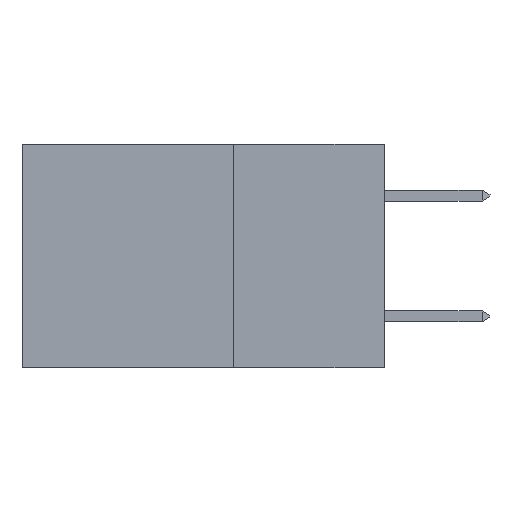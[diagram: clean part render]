
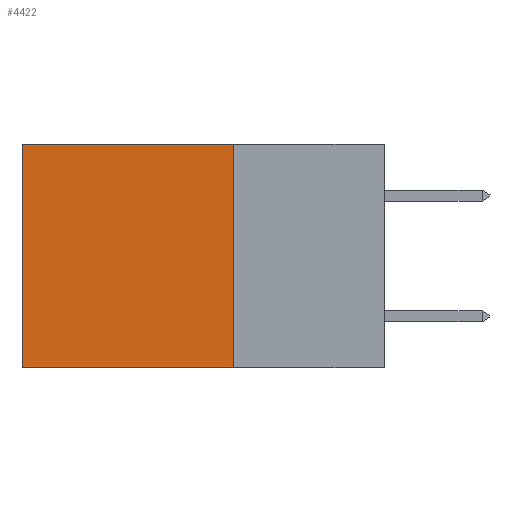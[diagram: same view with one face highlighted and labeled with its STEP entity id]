
A CAD part, left-side view. The second image highlights one B-rep face of the part: STEP entity #4422.
In plain terms, the highlighted planar face has unit normal (-1, 0, 0).
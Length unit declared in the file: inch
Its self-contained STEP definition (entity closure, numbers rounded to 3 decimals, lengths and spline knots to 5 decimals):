
#232 = CARTESIAN_POINT ( 'NONE',  ( 0.2875, 0.25, -0.37 ) ) ;
#830 = CARTESIAN_POINT ( 'NONE',  ( 0.2875, 0.6, 0. ) ) ;
#1557 = LINE ( 'NONE', #14088, #9302 ) ;
#1835 = EDGE_CURVE ( 'NONE', #6135, #8410, #2078, .T. ) ;
#2078 = LINE ( 'NONE', #830, #11527 ) ;
#2556 = ORIENTED_EDGE ( 'NONE', *, *, #1835, .T. ) ;
#2868 = DIRECTION ( 'NONE',  ( 0., 0., -1. ) ) ;
#3298 = ORIENTED_EDGE ( 'NONE', *, *, #4329, .F. ) ;
#4329 = EDGE_CURVE ( 'NONE', #14546, #8410, #8796, .T. ) ;
#4339 = CARTESIAN_POINT ( 'NONE',  ( 0.2875, 0.6, 0. ) ) ;
#4422 = ADVANCED_FACE ( 'NONE', ( #13824 ), #9104, .F. ) ;
#5185 = EDGE_CURVE ( 'NONE', #7229, #6135, #10296, .T. ) ;
#5516 = VECTOR ( 'NONE', #15006, 39.37008 ) ;
#5910 = CARTESIAN_POINT ( 'NONE',  ( 0.2875, 0.25, -0.37 ) ) ;
#6135 = VERTEX_POINT ( 'NONE', #4339 ) ;
#6553 = DIRECTION ( 'NONE',  ( 1., 0., 0. ) ) ;
#6693 = DIRECTION ( 'NONE',  ( 0., 0., -1. ) ) ;
#7088 = DIRECTION ( 'NONE',  ( 0., 0., -1. ) ) ;
#7229 = VERTEX_POINT ( 'NONE', #13575 ) ;
#7276 = ORIENTED_EDGE ( 'NONE', *, *, #11854, .F. ) ;
#8410 = VERTEX_POINT ( 'NONE', #12896 ) ;
#8796 = LINE ( 'NONE', #232, #5516 ) ;
#9104 = PLANE ( 'NONE',  #15269 ) ;
#9302 = VECTOR ( 'NONE', #6693, 39.37008 ) ;
#10137 = CARTESIAN_POINT ( 'NONE',  ( 0.2875, 0.25, 0. ) ) ;
#10296 = LINE ( 'NONE', #15114, #15608 ) ;
#11527 = VECTOR ( 'NONE', #7088, 39.37008 ) ;
#11826 = EDGE_LOOP ( 'NONE', ( #2556, #3298, #7276, #12595 ) ) ;
#11854 = EDGE_CURVE ( 'NONE', #7229, #14546, #1557, .T. ) ;
#12595 = ORIENTED_EDGE ( 'NONE', *, *, #5185, .T. ) ;
#12644 = DIRECTION ( 'NONE',  ( 0., 1., 0. ) ) ;
#12896 = CARTESIAN_POINT ( 'NONE',  ( 0.2875, 0.6, -0.37 ) ) ;
#13575 = CARTESIAN_POINT ( 'NONE',  ( 0.2875, 0.25, 0. ) ) ;
#13824 = FACE_OUTER_BOUND ( 'NONE', #11826, .T. ) ;
#14088 = CARTESIAN_POINT ( 'NONE',  ( 0.2875, 0.25, 0. ) ) ;
#14546 = VERTEX_POINT ( 'NONE', #5910 ) ;
#15006 = DIRECTION ( 'NONE',  ( 0., 1., 0. ) ) ;
#15114 = CARTESIAN_POINT ( 'NONE',  ( 0.2875, 0.25, 0. ) ) ;
#15269 = AXIS2_PLACEMENT_3D ( 'NONE', #10137, #6553, #2868 ) ;
#15608 = VECTOR ( 'NONE', #12644, 39.37008 ) ;
